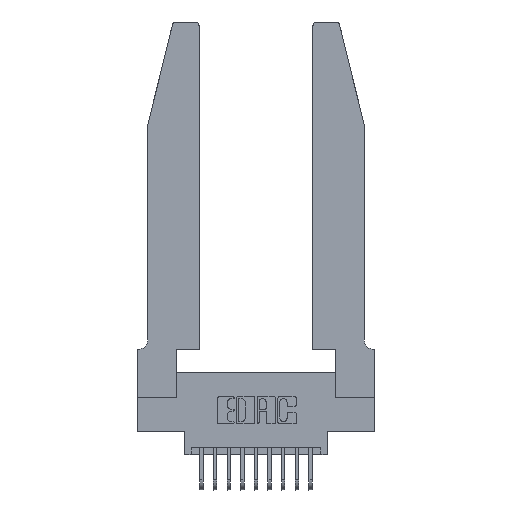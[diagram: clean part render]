
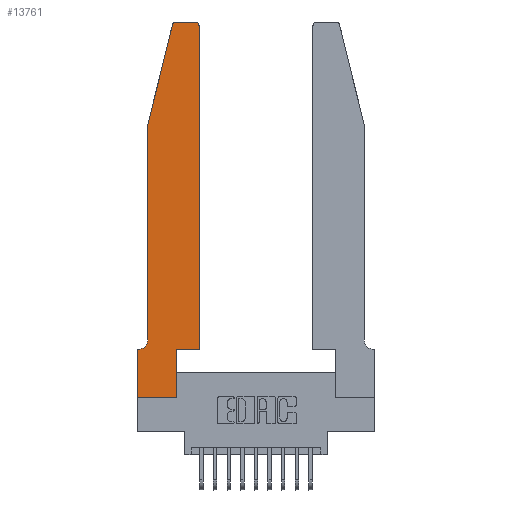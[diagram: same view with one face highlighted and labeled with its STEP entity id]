
A CAD part, top view. The second image highlights one B-rep face of the part: STEP entity #13761.
In plain terms, the highlighted planar face has unit normal (0, 0, 1).
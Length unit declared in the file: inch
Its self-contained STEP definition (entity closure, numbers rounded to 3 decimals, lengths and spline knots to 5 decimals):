
#56 = DIRECTION ( 'NONE',  ( 0., 1., 0. ) ) ;
#231 = ORIENTED_EDGE ( 'NONE', *, *, #17315, .T. ) ;
#374 = AXIS2_PLACEMENT_3D ( 'NONE', #6855, #16604, #16495 ) ;
#425 = LINE ( 'NONE', #17970, #3923 ) ;
#862 = DIRECTION ( 'NONE',  ( -1., 0., 0. ) ) ;
#1237 = AXIS2_PLACEMENT_3D ( 'NONE', #16967, #12794, #1793 ) ;
#1476 = AXIS2_PLACEMENT_3D ( 'NONE', #13032, #11592, #17236 ) ;
#1500 = CARTESIAN_POINT ( 'NONE',  ( 0.0755, 0.42, 0.37 ) ) ;
#1534 = VERTEX_POINT ( 'NONE', #9834 ) ;
#1793 = DIRECTION ( 'NONE',  ( 1., 0., 0. ) ) ;
#1976 = VERTEX_POINT ( 'NONE', #13676 ) ;
#2258 = CARTESIAN_POINT ( 'NONE',  ( 0.2865, 0.35, 0.37 ) ) ;
#2411 = LINE ( 'NONE', #16250, #7893 ) ;
#2443 = CARTESIAN_POINT ( 'NONE',  ( 0.2605, 2.75, 0.37 ) ) ;
#2873 = DIRECTION ( 'NONE',  ( 0., 0., -1. ) ) ;
#2913 = VERTEX_POINT ( 'NONE', #4190 ) ;
#2976 = CIRCLE ( 'NONE', #4895, 0.07 ) ;
#3212 = VERTEX_POINT ( 'NONE', #2258 ) ;
#3829 = VERTEX_POINT ( 'NONE', #7518 ) ;
#3923 = VECTOR ( 'NONE', #5615, 39.37008 ) ;
#4071 = VERTEX_POINT ( 'NONE', #17852 ) ;
#4088 = VERTEX_POINT ( 'NONE', #5256 ) ;
#4190 = CARTESIAN_POINT ( 'NONE',  ( 0.25487, 2.72718, 0.37 ) ) ;
#4473 = EDGE_CURVE ( 'NONE', #4088, #2913, #8591, .T. ) ;
#4729 = DIRECTION ( 'NONE',  ( -1., 0., 0. ) ) ;
#4895 = AXIS2_PLACEMENT_3D ( 'NONE', #6109, #2873, #17140 ) ;
#5011 = EDGE_CURVE ( 'NONE', #6428, #7793, #13561, .T. ) ;
#5256 = CARTESIAN_POINT ( 'NONE',  ( 0.284, 2.75, 0.37 ) ) ;
#5406 = CARTESIAN_POINT ( 'NONE',  ( 0.4505, 0.35, 0.37 ) ) ;
#5487 = VERTEX_POINT ( 'NONE', #9869 ) ;
#5615 = DIRECTION ( 'NONE',  ( 0., -1., 0. ) ) ;
#5687 = CARTESIAN_POINT ( 'NONE',  ( 0., 0.35, 0.37 ) ) ;
#5724 = VECTOR ( 'NONE', #13250, 39.37008 ) ;
#5805 = ORIENTED_EDGE ( 'NONE', *, *, #16891, .T. ) ;
#6109 = CARTESIAN_POINT ( 'NONE',  ( 0.0055, 0.42, 0.37 ) ) ;
#6428 = VERTEX_POINT ( 'NONE', #11242 ) ;
#6548 = DIRECTION ( 'NONE',  ( 0., 1., 0. ) ) ;
#6613 = ORIENTED_EDGE ( 'NONE', *, *, #14323, .T. ) ;
#6855 = CARTESIAN_POINT ( 'NONE',  ( 0.4205, 2.72, 0.37 ) ) ;
#7216 = PLANE ( 'NONE',  #1237 ) ;
#7518 = CARTESIAN_POINT ( 'NONE',  ( 0.4505, 0.35, 0.37 ) ) ;
#7793 = VERTEX_POINT ( 'NONE', #5687 ) ;
#7850 = LINE ( 'NONE', #11907, #15528 ) ;
#7893 = VECTOR ( 'NONE', #6548, 39.37008 ) ;
#8034 = EDGE_CURVE ( 'NONE', #14183, #1976, #12789, .T. ) ;
#8132 = ORIENTED_EDGE ( 'NONE', *, *, #5011, .T. ) ;
#8306 = CARTESIAN_POINT ( 'NONE',  ( 0.4505, 2.72, 0.37 ) ) ;
#8442 = LINE ( 'NONE', #9720, #13214 ) ;
#8543 = EDGE_LOOP ( 'NONE', ( #5805, #10832, #13556, #13067, #6613, #8132, #231, #15972, #12798, #14247, #12196, #9499 ) ) ;
#8591 = CIRCLE ( 'NONE', #1476, 0.03 ) ;
#9499 = ORIENTED_EDGE ( 'NONE', *, *, #8034, .T. ) ;
#9720 = CARTESIAN_POINT ( 'NONE',  ( 0., 0., 0.37 ) ) ;
#9811 = DIRECTION ( 'NONE',  ( 1., 0., 0. ) ) ;
#9834 = CARTESIAN_POINT ( 'NONE',  ( 0.2865, 0., 0.37 ) ) ;
#9869 = CARTESIAN_POINT ( 'NONE',  ( 0., 0., 0.37 ) ) ;
#10057 = VECTOR ( 'NONE', #56, 39.37008 ) ;
#10754 = LINE ( 'NONE', #11858, #5724 ) ;
#10832 = ORIENTED_EDGE ( 'NONE', *, *, #4473, .T. ) ;
#11074 = CARTESIAN_POINT ( 'NONE',  ( 0.4505, 0.35, 0.37 ) ) ;
#11127 = LINE ( 'NONE', #5406, #15476 ) ;
#11143 = DIRECTION ( 'NONE',  ( 1., 0., 0. ) ) ;
#11242 = CARTESIAN_POINT ( 'NONE',  ( 0.0055, 0.35, 0.37 ) ) ;
#11592 = DIRECTION ( 'NONE',  ( 0., 0., 1. ) ) ;
#11858 = CARTESIAN_POINT ( 'NONE',  ( 0.0755, 2., 0.37 ) ) ;
#11907 = CARTESIAN_POINT ( 'NONE',  ( 0., 0., 0.37 ) ) ;
#12053 = LINE ( 'NONE', #2443, #14879 ) ;
#12196 = ORIENTED_EDGE ( 'NONE', *, *, #17655, .T. ) ;
#12789 = CIRCLE ( 'NONE', #374, 0.03 ) ;
#12794 = DIRECTION ( 'NONE',  ( 0., 0., 1. ) ) ;
#12798 = ORIENTED_EDGE ( 'NONE', *, *, #16838, .T. ) ;
#12956 = EDGE_CURVE ( 'NONE', #3212, #3829, #11127, .T. ) ;
#13032 = CARTESIAN_POINT ( 'NONE',  ( 0.284, 2.72, 0.37 ) ) ;
#13067 = ORIENTED_EDGE ( 'NONE', *, *, #17585, .T. ) ;
#13214 = VECTOR ( 'NONE', #11143, 39.37008 ) ;
#13250 = DIRECTION ( 'NONE',  ( -0.239, -0.971, 0. ) ) ;
#13267 = CARTESIAN_POINT ( 'NONE',  ( 0.0755, 0.35, 0.37 ) ) ;
#13474 = DIRECTION ( 'NONE',  ( 0., -1., 0. ) ) ;
#13556 = ORIENTED_EDGE ( 'NONE', *, *, #16569, .T. ) ;
#13561 = LINE ( 'NONE', #13267, #14021 ) ;
#13619 = VERTEX_POINT ( 'NONE', #1500 ) ;
#13676 = CARTESIAN_POINT ( 'NONE',  ( 0.4205, 2.75, 0.37 ) ) ;
#13761 = ADVANCED_FACE ( 'NONE', ( #17809 ), #7216, .T. ) ;
#14021 = VECTOR ( 'NONE', #4729, 39.37008 ) ;
#14183 = VERTEX_POINT ( 'NONE', #8306 ) ;
#14191 = EDGE_CURVE ( 'NONE', #5487, #1534, #8442, .T. ) ;
#14247 = ORIENTED_EDGE ( 'NONE', *, *, #12956, .T. ) ;
#14323 = EDGE_CURVE ( 'NONE', #13619, #6428, #2976, .T. ) ;
#14879 = VECTOR ( 'NONE', #862, 39.37008 ) ;
#15476 = VECTOR ( 'NONE', #9811, 39.37008 ) ;
#15528 = VECTOR ( 'NONE', #13474, 39.37008 ) ;
#15972 = ORIENTED_EDGE ( 'NONE', *, *, #14191, .T. ) ;
#16250 = CARTESIAN_POINT ( 'NONE',  ( 0.2865, 0.35, 0.37 ) ) ;
#16495 = DIRECTION ( 'NONE',  ( 1., 0., 0. ) ) ;
#16569 = EDGE_CURVE ( 'NONE', #2913, #4071, #10754, .T. ) ;
#16604 = DIRECTION ( 'NONE',  ( 0., 0., 1. ) ) ;
#16802 = LINE ( 'NONE', #11074, #10057 ) ;
#16838 = EDGE_CURVE ( 'NONE', #1534, #3212, #2411, .T. ) ;
#16891 = EDGE_CURVE ( 'NONE', #1976, #4088, #12053, .T. ) ;
#16967 = CARTESIAN_POINT ( 'NONE',  ( 0., 0.35, 0.37 ) ) ;
#17140 = DIRECTION ( 'NONE',  ( -1., 0., 0. ) ) ;
#17236 = DIRECTION ( 'NONE',  ( 1., 0., 0. ) ) ;
#17315 = EDGE_CURVE ( 'NONE', #7793, #5487, #7850, .T. ) ;
#17585 = EDGE_CURVE ( 'NONE', #4071, #13619, #425, .T. ) ;
#17655 = EDGE_CURVE ( 'NONE', #3829, #14183, #16802, .T. ) ;
#17809 = FACE_OUTER_BOUND ( 'NONE', #8543, .T. ) ;
#17852 = CARTESIAN_POINT ( 'NONE',  ( 0.0755, 2., 0.37 ) ) ;
#17970 = CARTESIAN_POINT ( 'NONE',  ( 0.0755, 2., 0.37 ) ) ;
